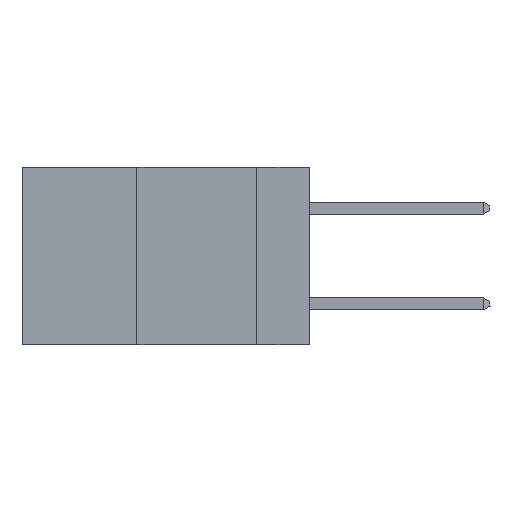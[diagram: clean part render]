
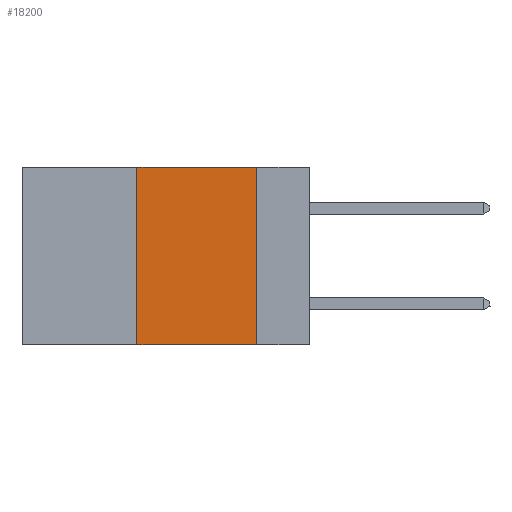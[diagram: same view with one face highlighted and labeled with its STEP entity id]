
A CAD part, left-side view. The second image highlights one B-rep face of the part: STEP entity #18200.
In plain terms, the highlighted planar face has unit normal (-1, 0, 0).
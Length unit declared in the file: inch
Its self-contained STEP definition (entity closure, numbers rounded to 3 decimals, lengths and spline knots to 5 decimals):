
#532 = FACE_OUTER_BOUND ( 'NONE', #17679, .T. ) ;
#878 = CARTESIAN_POINT ( 'NONE',  ( 0., 0.6, 0. ) ) ;
#1181 = VECTOR ( 'NONE', #17607, 39.37008 ) ;
#1808 = CARTESIAN_POINT ( 'NONE',  ( 0., 0.6, -0.37 ) ) ;
#3590 = LINE ( 'NONE', #1808, #7675 ) ;
#4031 = DIRECTION ( 'NONE',  ( 0., 0., -1. ) ) ;
#4648 = LINE ( 'NONE', #878, #13516 ) ;
#5639 = CARTESIAN_POINT ( 'NONE',  ( 0., 0.6, 0. ) ) ;
#5831 = ORIENTED_EDGE ( 'NONE', *, *, #14623, .F. ) ;
#5858 = CARTESIAN_POINT ( 'NONE',  ( 0., 0.11, 0. ) ) ;
#6970 = DIRECTION ( 'NONE',  ( 0., 0., -1. ) ) ;
#7675 = VECTOR ( 'NONE', #14273, 39.37008 ) ;
#8295 = CARTESIAN_POINT ( 'NONE',  ( 0., 0.11, -0.37 ) ) ;
#8874 = PLANE ( 'NONE',  #12212 ) ;
#9167 = VECTOR ( 'NONE', #6970, 39.37008 ) ;
#10877 = VERTEX_POINT ( 'NONE', #17216 ) ;
#11304 = VERTEX_POINT ( 'NONE', #8295 ) ;
#12212 = AXIS2_PLACEMENT_3D ( 'NONE', #5639, #13225, #4031 ) ;
#12903 = CARTESIAN_POINT ( 'NONE',  ( 0., 0.36, 0. ) ) ;
#13225 = DIRECTION ( 'NONE',  ( 1., 0., 0. ) ) ;
#13238 = LINE ( 'NONE', #5858, #9167 ) ;
#13516 = VECTOR ( 'NONE', #13628, 39.37008 ) ;
#13569 = EDGE_CURVE ( 'NONE', #10877, #11304, #13238, .T. ) ;
#13628 = DIRECTION ( 'NONE',  ( 0., -1., 0. ) ) ;
#13830 = VERTEX_POINT ( 'NONE', #18000 ) ;
#14273 = DIRECTION ( 'NONE',  ( 0., -1., 0. ) ) ;
#14623 = EDGE_CURVE ( 'NONE', #18249, #13830, #15637, .T. ) ;
#14780 = CARTESIAN_POINT ( 'NONE',  ( 0., 0.36, -0.37 ) ) ;
#15209 = EDGE_CURVE ( 'NONE', #18249, #11304, #3590, .T. ) ;
#15637 = LINE ( 'NONE', #12903, #1181 ) ;
#17216 = CARTESIAN_POINT ( 'NONE',  ( 0., 0.11, 0. ) ) ;
#17607 = DIRECTION ( 'NONE',  ( 0., 0., 1. ) ) ;
#17679 = EDGE_LOOP ( 'NONE', ( #17773, #19490, #5831, #18605 ) ) ;
#17773 = ORIENTED_EDGE ( 'NONE', *, *, #13569, .F. ) ;
#18000 = CARTESIAN_POINT ( 'NONE',  ( 0., 0.36, 0. ) ) ;
#18200 = ADVANCED_FACE ( 'NONE', ( #532 ), #8874, .F. ) ;
#18249 = VERTEX_POINT ( 'NONE', #14780 ) ;
#18605 = ORIENTED_EDGE ( 'NONE', *, *, #15209, .T. ) ;
#18920 = EDGE_CURVE ( 'NONE', #13830, #10877, #4648, .T. ) ;
#19490 = ORIENTED_EDGE ( 'NONE', *, *, #18920, .F. ) ;
